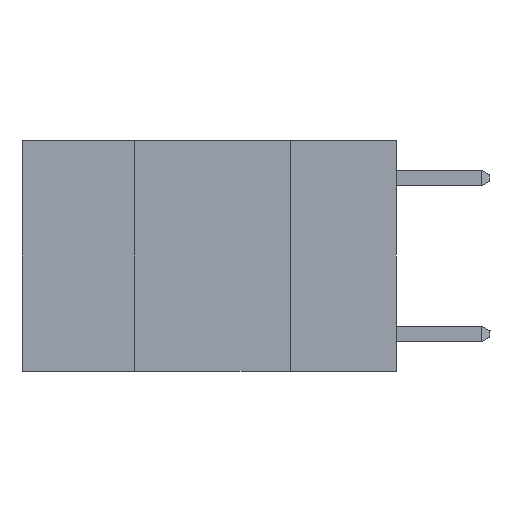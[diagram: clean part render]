
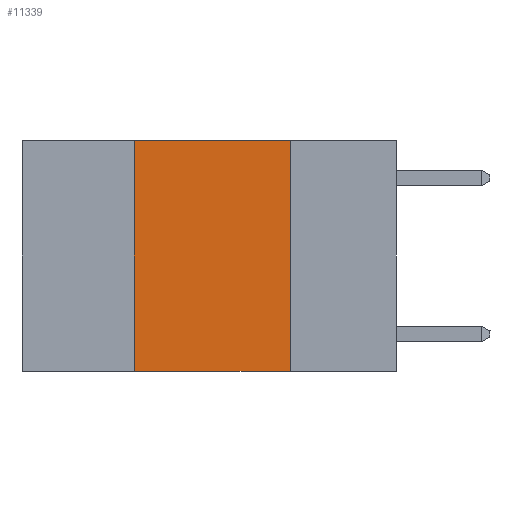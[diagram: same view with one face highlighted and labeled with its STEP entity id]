
A CAD part, left-side view. The second image highlights one B-rep face of the part: STEP entity #11339.
In plain terms, the highlighted planar face has unit normal (-1, 0, 0).
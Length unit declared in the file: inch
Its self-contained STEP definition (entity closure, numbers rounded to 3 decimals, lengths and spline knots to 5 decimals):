
#549 = DIRECTION ( 'NONE',  ( 0., 0., -1. ) ) ;
#622 = DIRECTION ( 'NONE',  ( 0., -1., 0. ) ) ;
#836 = EDGE_CURVE ( 'NONE', #11800, #15656, #26075, .T. ) ;
#1802 = EDGE_LOOP ( 'NONE', ( #10273, #12790, #22169, #4743 ) ) ;
#2122 = DIRECTION ( 'NONE',  ( 0., 0., -1. ) ) ;
#3946 = CARTESIAN_POINT ( 'NONE',  ( 0., 0.17, -0.37 ) ) ;
#4743 = ORIENTED_EDGE ( 'NONE', *, *, #22801, .T. ) ;
#4972 = CARTESIAN_POINT ( 'NONE',  ( 0., 0.6, -0.37 ) ) ;
#5923 = PLANE ( 'NONE',  #19134 ) ;
#8453 = DIRECTION ( 'NONE',  ( 1., 0., 0. ) ) ;
#9256 = EDGE_CURVE ( 'NONE', #15656, #13077, #11305, .T. ) ;
#9545 = VECTOR ( 'NONE', #549, 39.37008 ) ;
#10273 = ORIENTED_EDGE ( 'NONE', *, *, #19251, .F. ) ;
#11165 = DIRECTION ( 'NONE',  ( 0., -1., 0. ) ) ;
#11167 = DIRECTION ( 'NONE',  ( 0., 0., 1. ) ) ;
#11305 = LINE ( 'NONE', #24399, #19991 ) ;
#11339 = ADVANCED_FACE ( 'NONE', ( #27289 ), #5923, .F. ) ;
#11800 = VERTEX_POINT ( 'NONE', #25959 ) ;
#12426 = VECTOR ( 'NONE', #622, 39.37008 ) ;
#12790 = ORIENTED_EDGE ( 'NONE', *, *, #9256, .F. ) ;
#13077 = VERTEX_POINT ( 'NONE', #20549 ) ;
#13290 = CARTESIAN_POINT ( 'NONE',  ( 0., 0.42, 0. ) ) ;
#15059 = CARTESIAN_POINT ( 'NONE',  ( 0., 0.6, 0. ) ) ;
#15580 = VERTEX_POINT ( 'NONE', #3946 ) ;
#15656 = VERTEX_POINT ( 'NONE', #18988 ) ;
#17680 = LINE ( 'NONE', #24439, #9545 ) ;
#18988 = CARTESIAN_POINT ( 'NONE',  ( 0., 0.42, 0. ) ) ;
#19134 = AXIS2_PLACEMENT_3D ( 'NONE', #15059, #8453, #2122 ) ;
#19251 = EDGE_CURVE ( 'NONE', #13077, #15580, #17680, .T. ) ;
#19991 = VECTOR ( 'NONE', #11165, 39.37008 ) ;
#20549 = CARTESIAN_POINT ( 'NONE',  ( 0., 0.17, 0. ) ) ;
#22169 = ORIENTED_EDGE ( 'NONE', *, *, #836, .F. ) ;
#22801 = EDGE_CURVE ( 'NONE', #11800, #15580, #24509, .T. ) ;
#24399 = CARTESIAN_POINT ( 'NONE',  ( 0., 0.6, 0. ) ) ;
#24439 = CARTESIAN_POINT ( 'NONE',  ( 0., 0.17, 0. ) ) ;
#24509 = LINE ( 'NONE', #4972, #12426 ) ;
#25959 = CARTESIAN_POINT ( 'NONE',  ( 0., 0.42, -0.37 ) ) ;
#26075 = LINE ( 'NONE', #13290, #26326 ) ;
#26326 = VECTOR ( 'NONE', #11167, 39.37008 ) ;
#27289 = FACE_OUTER_BOUND ( 'NONE', #1802, .T. ) ;
